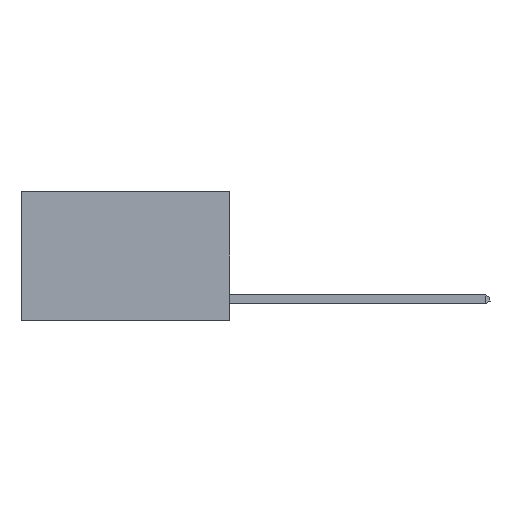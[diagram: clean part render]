
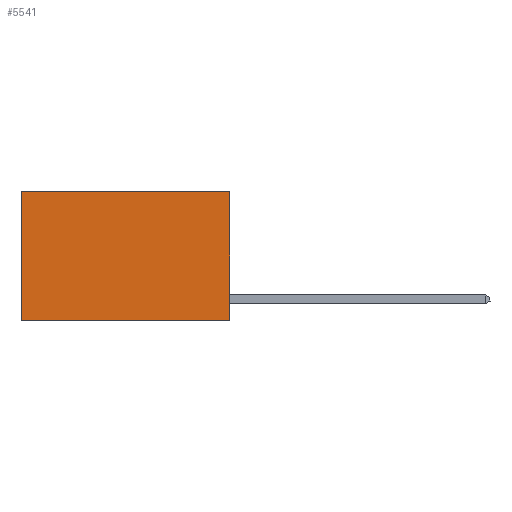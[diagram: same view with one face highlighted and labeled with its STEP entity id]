
A CAD part, left-side view. The second image highlights one B-rep face of the part: STEP entity #5541.
In plain terms, the highlighted planar face has unit normal (-1, 0, 0).
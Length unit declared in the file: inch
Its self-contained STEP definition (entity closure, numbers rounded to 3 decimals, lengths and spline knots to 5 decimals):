
#876 = ORIENTED_EDGE ( 'NONE', *, *, #6868, .F. ) ;
#1074 = CARTESIAN_POINT ( 'NONE',  ( 0.2625, 0.6, 0. ) ) ;
#1920 = DIRECTION ( 'NONE',  ( 0., 0., -1. ) ) ;
#4565 = CARTESIAN_POINT ( 'NONE',  ( 0.2625, 0., 0. ) ) ;
#5292 = CARTESIAN_POINT ( 'NONE',  ( 0.2625, 0., -0.37 ) ) ;
#5541 = ADVANCED_FACE ( 'NONE', ( #6309 ), #14209, .F. ) ;
#5631 = CARTESIAN_POINT ( 'NONE',  ( 0.2625, 0., 0. ) ) ;
#6261 = EDGE_CURVE ( 'NONE', #6428, #14121, #7175, .T. ) ;
#6309 = FACE_OUTER_BOUND ( 'NONE', #15543, .T. ) ;
#6379 = VECTOR ( 'NONE', #1920, 39.37008 ) ;
#6428 = VERTEX_POINT ( 'NONE', #1074 ) ;
#6587 = CARTESIAN_POINT ( 'NONE',  ( 0.2625, 0., -0.37 ) ) ;
#6868 = EDGE_CURVE ( 'NONE', #18848, #14121, #8036, .T. ) ;
#7175 = LINE ( 'NONE', #16713, #12362 ) ;
#7429 = CARTESIAN_POINT ( 'NONE',  ( 0.2625, 0., 0. ) ) ;
#8036 = LINE ( 'NONE', #5292, #9835 ) ;
#8274 = ORIENTED_EDGE ( 'NONE', *, *, #8738, .F. ) ;
#8738 = EDGE_CURVE ( 'NONE', #15753, #18848, #19120, .T. ) ;
#9416 = DIRECTION ( 'NONE',  ( 0., 0., -1. ) ) ;
#9835 = VECTOR ( 'NONE', #12309, 39.37008 ) ;
#11752 = DIRECTION ( 'NONE',  ( 0., 0., -1. ) ) ;
#11968 = ORIENTED_EDGE ( 'NONE', *, *, #6261, .T. ) ;
#12214 = LINE ( 'NONE', #7429, #20430 ) ;
#12309 = DIRECTION ( 'NONE',  ( 0., 1., 0. ) ) ;
#12362 = VECTOR ( 'NONE', #11752, 39.37008 ) ;
#12430 = DIRECTION ( 'NONE',  ( 1., 0., 0. ) ) ;
#12687 = AXIS2_PLACEMENT_3D ( 'NONE', #4565, #12430, #9416 ) ;
#13759 = DIRECTION ( 'NONE',  ( 0., 1., 0. ) ) ;
#14121 = VERTEX_POINT ( 'NONE', #17976 ) ;
#14209 = PLANE ( 'NONE',  #12687 ) ;
#14896 = ORIENTED_EDGE ( 'NONE', *, *, #15309, .T. ) ;
#15309 = EDGE_CURVE ( 'NONE', #15753, #6428, #12214, .T. ) ;
#15543 = EDGE_LOOP ( 'NONE', ( #11968, #876, #8274, #14896 ) ) ;
#15753 = VERTEX_POINT ( 'NONE', #5631 ) ;
#16015 = CARTESIAN_POINT ( 'NONE',  ( 0.2625, 0., 0. ) ) ;
#16713 = CARTESIAN_POINT ( 'NONE',  ( 0.2625, 0.6, 0. ) ) ;
#17976 = CARTESIAN_POINT ( 'NONE',  ( 0.2625, 0.6, -0.37 ) ) ;
#18848 = VERTEX_POINT ( 'NONE', #6587 ) ;
#19120 = LINE ( 'NONE', #16015, #6379 ) ;
#20430 = VECTOR ( 'NONE', #13759, 39.37008 ) ;
